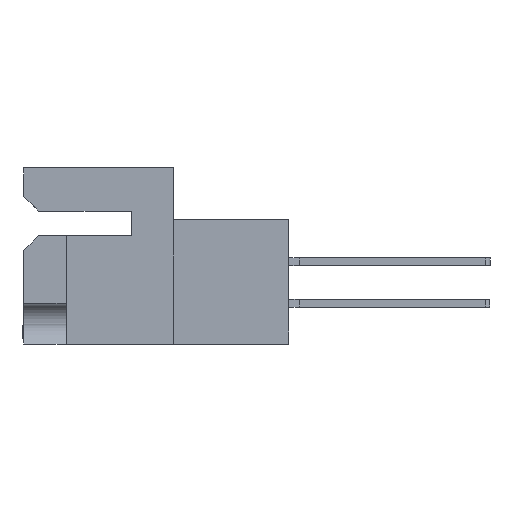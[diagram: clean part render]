
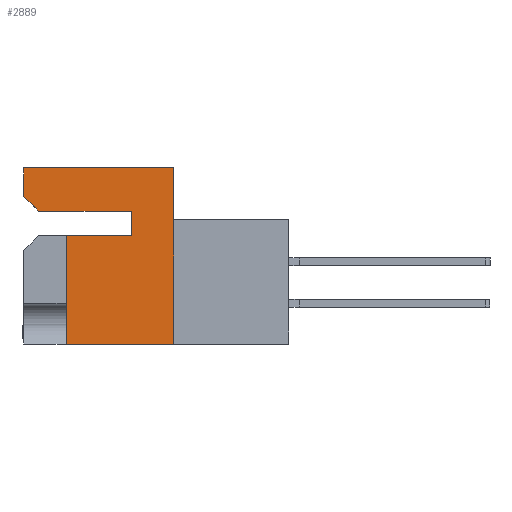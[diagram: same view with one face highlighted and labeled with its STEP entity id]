
A CAD part, left-side view. The second image highlights one B-rep face of the part: STEP entity #2889.
In plain terms, the highlighted planar face has unit normal (-1, 0, 0).
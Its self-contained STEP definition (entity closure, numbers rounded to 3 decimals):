
#237 = DIRECTION ( 'NONE',  ( 0., 1., 0. ) ) ;
#678 = LINE ( 'NONE', #4713, #24045 ) ;
#1284 = DIRECTION ( 'NONE',  ( 0., 0., 1. ) ) ;
#1419 = VERTEX_POINT ( 'NONE', #1723 ) ;
#1613 = VECTOR ( 'NONE', #14985, 1000. ) ;
#1723 = CARTESIAN_POINT ( 'NONE',  ( 0., 8.255, -13.487 ) ) ;
#2080 = ORIENTED_EDGE ( 'NONE', *, *, #15239, .F. ) ;
#2118 = CARTESIAN_POINT ( 'NONE',  ( 0., 11.506, -13.487 ) ) ;
#2410 = VERTEX_POINT ( 'NONE', #19716 ) ;
#2889 = ADVANCED_FACE ( 'NONE', ( #22447 ), #24185, .F. ) ;
#3482 = LINE ( 'NONE', #5006, #28594 ) ;
#4081 = LINE ( 'NONE', #13228, #29545 ) ;
#4095 = CARTESIAN_POINT ( 'NONE',  ( 0., 11.506, 0. ) ) ;
#4713 = CARTESIAN_POINT ( 'NONE',  ( 0., 10.363, -3.302 ) ) ;
#5006 = CARTESIAN_POINT ( 'NONE',  ( 0., 0., -3.302 ) ) ;
#5539 = DIRECTION ( 'NONE',  ( 0., -1., 0. ) ) ;
#5778 = EDGE_CURVE ( 'NONE', #1419, #18352, #27520, .T. ) ;
#5978 = VECTOR ( 'NONE', #5539, 1000. ) ;
#6001 = LINE ( 'NONE', #4095, #26085 ) ;
#6161 = LINE ( 'NONE', #2118, #11486 ) ;
#6768 = VERTEX_POINT ( 'NONE', #27001 ) ;
#8234 = ORIENTED_EDGE ( 'NONE', *, *, #14802, .F. ) ;
#8496 = ORIENTED_EDGE ( 'NONE', *, *, #21210, .F. ) ;
#8571 = VERTEX_POINT ( 'NONE', #25508 ) ;
#8840 = DIRECTION ( 'NONE',  ( 0., 1., 0. ) ) ;
#8923 = CARTESIAN_POINT ( 'NONE',  ( 0., 0., 0. ) ) ;
#9923 = CARTESIAN_POINT ( 'NONE',  ( 0., 0., -5.182 ) ) ;
#10081 = ORIENTED_EDGE ( 'NONE', *, *, #24017, .F. ) ;
#10893 = EDGE_CURVE ( 'NONE', #2410, #26242, #6161, .T. ) ;
#11486 = VECTOR ( 'NONE', #20758, 1000. ) ;
#11670 = LINE ( 'NONE', #9923, #5978 ) ;
#11695 = EDGE_CURVE ( 'NONE', #2410, #6768, #678, .T. ) ;
#12197 = ORIENTED_EDGE ( 'NONE', *, *, #10893, .F. ) ;
#13228 = CARTESIAN_POINT ( 'NONE',  ( 0., -8.814, -13.487 ) ) ;
#13650 = EDGE_LOOP ( 'NONE', ( #19015, #10081, #17402, #12197, #15054, #8234, #8496, #2080, #28516 ) ) ;
#14695 = EDGE_CURVE ( 'NONE', #26242, #15357, #6001, .T. ) ;
#14802 = EDGE_CURVE ( 'NONE', #28366, #6768, #3482, .T. ) ;
#14985 = DIRECTION ( 'NONE',  ( 0., 0., 1. ) ) ;
#15015 = CARTESIAN_POINT ( 'NONE',  ( 0., 8.255, -5.182 ) ) ;
#15054 = ORIENTED_EDGE ( 'NONE', *, *, #11695, .T. ) ;
#15239 = EDGE_CURVE ( 'NONE', #18352, #8571, #11670, .T. ) ;
#15357 = VERTEX_POINT ( 'NONE', #21369 ) ;
#15601 = AXIS2_PLACEMENT_3D ( 'NONE', #26311, #23876, #21972 ) ;
#15898 = DIRECTION ( 'NONE',  ( 0., -1., 0. ) ) ;
#16590 = LINE ( 'NONE', #8923, #20181 ) ;
#16855 = EDGE_CURVE ( 'NONE', #21138, #1419, #4081, .T. ) ;
#17402 = ORIENTED_EDGE ( 'NONE', *, *, #14695, .F. ) ;
#18238 = DIRECTION ( 'NONE',  ( 0., 0., -1. ) ) ;
#18352 = VERTEX_POINT ( 'NONE', #23906 ) ;
#19015 = ORIENTED_EDGE ( 'NONE', *, *, #16855, .F. ) ;
#19018 = CARTESIAN_POINT ( 'NONE',  ( 0., 3.251, -3.302 ) ) ;
#19716 = CARTESIAN_POINT ( 'NONE',  ( 0., 11.506, -2.159 ) ) ;
#20181 = VECTOR ( 'NONE', #18238, 1000. ) ;
#20758 = DIRECTION ( 'NONE',  ( 0., 0., 1. ) ) ;
#21131 = DIRECTION ( 'NONE',  ( 0., -0.707, -0.707 ) ) ;
#21138 = VERTEX_POINT ( 'NONE', #26252 ) ;
#21210 = EDGE_CURVE ( 'NONE', #8571, #28366, #28910, .T. ) ;
#21369 = CARTESIAN_POINT ( 'NONE',  ( 0., 0., 0. ) ) ;
#21428 = VECTOR ( 'NONE', #1284, 1000. ) ;
#21972 = DIRECTION ( 'NONE',  ( 0., 0., -1. ) ) ;
#22447 = FACE_OUTER_BOUND ( 'NONE', #13650, .T. ) ;
#23149 = CARTESIAN_POINT ( 'NONE',  ( 0., 11.506, 0. ) ) ;
#23876 = DIRECTION ( 'NONE',  ( 1., 0., 0. ) ) ;
#23906 = CARTESIAN_POINT ( 'NONE',  ( 0., 8.255, -5.182 ) ) ;
#24017 = EDGE_CURVE ( 'NONE', #15357, #21138, #16590, .T. ) ;
#24045 = VECTOR ( 'NONE', #21131, 1000. ) ;
#24185 = PLANE ( 'NONE',  #15601 ) ;
#25508 = CARTESIAN_POINT ( 'NONE',  ( 0., 3.251, -5.182 ) ) ;
#26085 = VECTOR ( 'NONE', #15898, 1000. ) ;
#26242 = VERTEX_POINT ( 'NONE', #23149 ) ;
#26252 = CARTESIAN_POINT ( 'NONE',  ( 0., 0., -13.487 ) ) ;
#26311 = CARTESIAN_POINT ( 'NONE',  ( 0., 0., 0. ) ) ;
#27001 = CARTESIAN_POINT ( 'NONE',  ( 0., 10.363, -3.302 ) ) ;
#27520 = LINE ( 'NONE', #15015, #21428 ) ;
#28366 = VERTEX_POINT ( 'NONE', #19018 ) ;
#28516 = ORIENTED_EDGE ( 'NONE', *, *, #5778, .F. ) ;
#28525 = CARTESIAN_POINT ( 'NONE',  ( 0., 3.251, -5.182 ) ) ;
#28594 = VECTOR ( 'NONE', #237, 1000. ) ;
#28910 = LINE ( 'NONE', #28525, #1613 ) ;
#29545 = VECTOR ( 'NONE', #8840, 1000. ) ;
